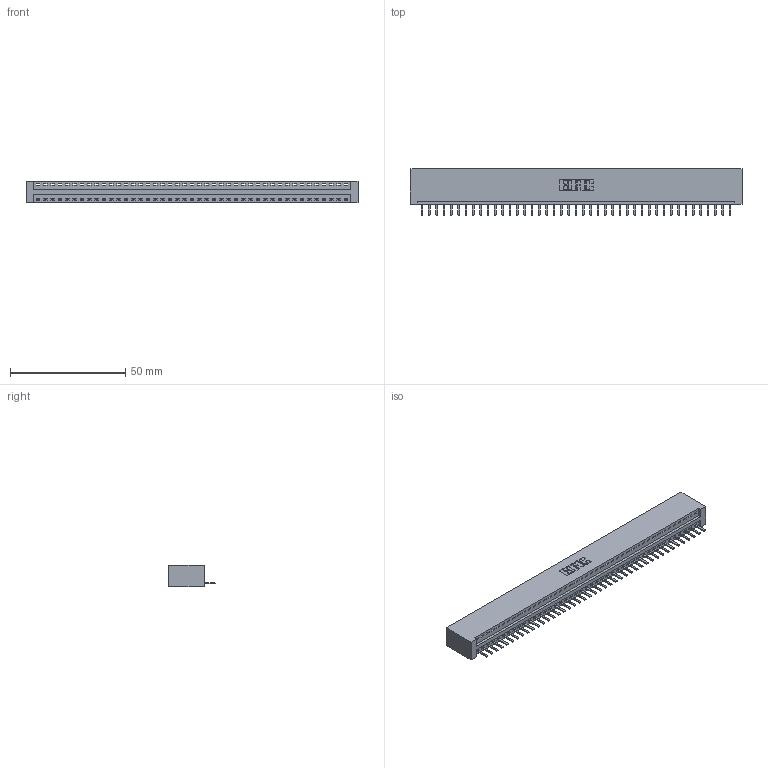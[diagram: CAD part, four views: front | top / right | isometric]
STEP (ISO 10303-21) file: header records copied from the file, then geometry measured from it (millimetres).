
FILE_DESCRIPTION (( 'STEP AP203' ), '1' );
FILE_NAME ('346-043-520-101.STEP', '2022-05-09T15:14:51', ( '' ), ( '' ), 'SwSTEP 2.0', 'SolidWorks 2020', '' );
FILE_SCHEMA (( 'CONFIG_CONTROL_DESIGN' ));
Length unit declared in the file: inch
Products named in the file (3): 346-043-520-101; 346 Part_No Mounting Lugs; 345-292-001_345-293-120
Assembly tree (44 placements, depth 2):
  346-043-520-101
    346 Part_No Mounting Lugs
    345-292-001_345-293-120  x43
Bounding box: 143.76 x 20.02 x 9.4 mm (x, y, z)
Volume: 14194 mm3; surface area: 17413.7 mm2
Topology: 44 solids, 44 shells, 2780 faces, 8217 edges, 5362 vertices
Faces by surface type: plane 1878, cylinder 902
Entity records: 26389 total; most frequent: CARTESIAN_POINT 4541, ORIENTED_EDGE 4506, DIRECTION 3987, EDGE_CURVE 2253, VECTOR 1953, LINE 1953, VERTEX_POINT 1498, AXIS2_PLACEMENT_3D 1017
